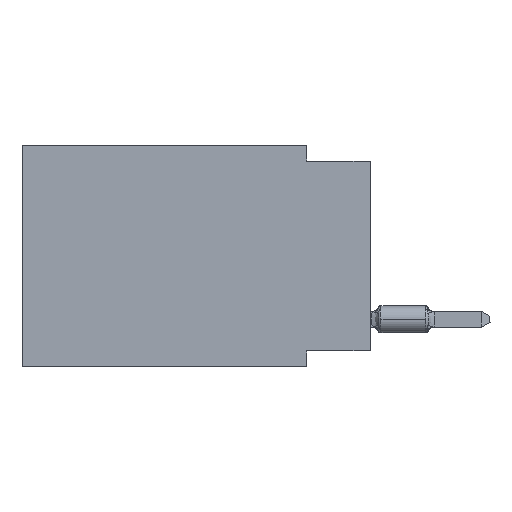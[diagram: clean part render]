
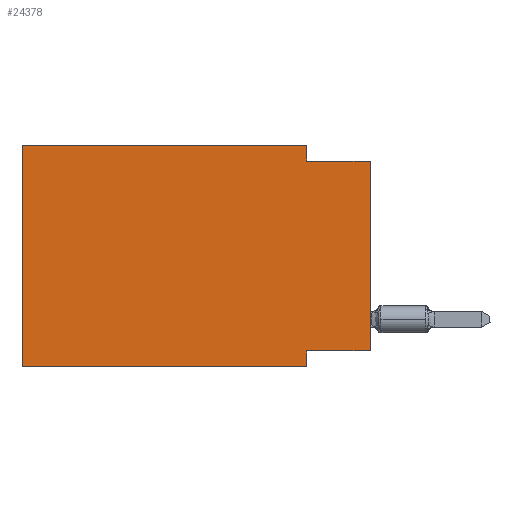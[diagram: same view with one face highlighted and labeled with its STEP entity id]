
A CAD part, left-side view. The second image highlights one B-rep face of the part: STEP entity #24378.
In plain terms, the highlighted planar face has unit normal (-1, 0, 0).
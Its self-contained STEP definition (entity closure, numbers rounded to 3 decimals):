
#668 = CARTESIAN_POINT ( 'NONE',  ( 0., 0., 0. ) ) ;
#763 = VECTOR ( 'NONE', #11287, 1000. ) ;
#2521 = CARTESIAN_POINT ( 'NONE',  ( 0., 2.54, -0.635 ) ) ;
#2656 = CARTESIAN_POINT ( 'NONE',  ( 0., 2.54, 0. ) ) ;
#3002 = DIRECTION ( 'NONE',  ( 0., 0., 1. ) ) ;
#3403 = DIRECTION ( 'NONE',  ( 0., -1., 0. ) ) ;
#3644 = EDGE_CURVE ( 'NONE', #13062, #7990, #9696, .T. ) ;
#3653 = LINE ( 'NONE', #25619, #9620 ) ;
#4362 = VERTEX_POINT ( 'NONE', #22403 ) ;
#4549 = DIRECTION ( 'NONE',  ( 0., 0., 1. ) ) ;
#5601 = LINE ( 'NONE', #14539, #17971 ) ;
#6176 = VERTEX_POINT ( 'NONE', #28338 ) ;
#6414 = DIRECTION ( 'NONE',  ( 0., -1., 0. ) ) ;
#6624 = LINE ( 'NONE', #9249, #17057 ) ;
#6654 = ORIENTED_EDGE ( 'NONE', *, *, #24984, .F. ) ;
#7820 = EDGE_CURVE ( 'NONE', #14424, #12782, #5601, .T. ) ;
#7990 = VERTEX_POINT ( 'NONE', #2521 ) ;
#9069 = CARTESIAN_POINT ( 'NONE',  ( 0., 13.97, 0. ) ) ;
#9249 = CARTESIAN_POINT ( 'NONE',  ( 0., 13.97, 0. ) ) ;
#9466 = LINE ( 'NONE', #668, #21795 ) ;
#9509 = ORIENTED_EDGE ( 'NONE', *, *, #7820, .F. ) ;
#9607 = EDGE_LOOP ( 'NONE', ( #22458, #11606, #20179, #6654, #10444, #12273, #9509, #18789 ) ) ;
#9620 = VECTOR ( 'NONE', #25482, 1000. ) ;
#9696 = LINE ( 'NONE', #2656, #17703 ) ;
#10444 = ORIENTED_EDGE ( 'NONE', *, *, #23944, .F. ) ;
#10953 = CARTESIAN_POINT ( 'NONE',  ( 0., 13.97, -8.89 ) ) ;
#11287 = DIRECTION ( 'NONE',  ( 0., 1., 0. ) ) ;
#11411 = DIRECTION ( 'NONE',  ( 1., 0., 0. ) ) ;
#11452 = DIRECTION ( 'NONE',  ( 0., 0., -1. ) ) ;
#11606 = ORIENTED_EDGE ( 'NONE', *, *, #23545, .F. ) ;
#12273 = ORIENTED_EDGE ( 'NONE', *, *, #27142, .T. ) ;
#12782 = VERTEX_POINT ( 'NONE', #22740 ) ;
#13062 = VERTEX_POINT ( 'NONE', #21847 ) ;
#13193 = CARTESIAN_POINT ( 'NONE',  ( 0., 0., -8.255 ) ) ;
#13339 = AXIS2_PLACEMENT_3D ( 'NONE', #9069, #11411, #20314 ) ;
#14209 = VERTEX_POINT ( 'NONE', #18851 ) ;
#14424 = VERTEX_POINT ( 'NONE', #16151 ) ;
#14539 = CARTESIAN_POINT ( 'NONE',  ( 0., 2.54, -8.89 ) ) ;
#14640 = VERTEX_POINT ( 'NONE', #24181 ) ;
#15621 = VECTOR ( 'NONE', #3403, 1000. ) ;
#16151 = CARTESIAN_POINT ( 'NONE',  ( 0., 2.54, -8.255 ) ) ;
#16248 = EDGE_CURVE ( 'NONE', #14209, #6176, #9466, .T. ) ;
#17057 = VECTOR ( 'NONE', #4549, 1000. ) ;
#17703 = VECTOR ( 'NONE', #11452, 1000. ) ;
#17771 = EDGE_CURVE ( 'NONE', #14209, #14424, #24301, .T. ) ;
#17971 = VECTOR ( 'NONE', #25512, 1000. ) ;
#18789 = ORIENTED_EDGE ( 'NONE', *, *, #17771, .F. ) ;
#18851 = CARTESIAN_POINT ( 'NONE',  ( 0., 0., -8.255 ) ) ;
#20171 = FACE_OUTER_BOUND ( 'NONE', #9607, .T. ) ;
#20179 = ORIENTED_EDGE ( 'NONE', *, *, #3644, .F. ) ;
#20314 = DIRECTION ( 'NONE',  ( 0., 0., -1. ) ) ;
#21795 = VECTOR ( 'NONE', #3002, 1000. ) ;
#21847 = CARTESIAN_POINT ( 'NONE',  ( 0., 2.54, 0. ) ) ;
#22403 = CARTESIAN_POINT ( 'NONE',  ( 0., 13.97, -8.89 ) ) ;
#22458 = ORIENTED_EDGE ( 'NONE', *, *, #16248, .T. ) ;
#22740 = CARTESIAN_POINT ( 'NONE',  ( 0., 2.54, -8.89 ) ) ;
#23545 = EDGE_CURVE ( 'NONE', #7990, #6176, #25211, .T. ) ;
#23944 = EDGE_CURVE ( 'NONE', #4362, #14640, #6624, .T. ) ;
#24181 = CARTESIAN_POINT ( 'NONE',  ( 0., 13.97, 0. ) ) ;
#24301 = LINE ( 'NONE', #13193, #763 ) ;
#24378 = ADVANCED_FACE ( 'NONE', ( #20171 ), #26897, .F. ) ;
#24984 = EDGE_CURVE ( 'NONE', #14640, #13062, #3653, .T. ) ;
#25211 = LINE ( 'NONE', #27686, #15621 ) ;
#25482 = DIRECTION ( 'NONE',  ( 0., -1., 0. ) ) ;
#25512 = DIRECTION ( 'NONE',  ( 0., 0., -1. ) ) ;
#25619 = CARTESIAN_POINT ( 'NONE',  ( 0., 13.97, 0. ) ) ;
#26447 = LINE ( 'NONE', #10953, #27068 ) ;
#26897 = PLANE ( 'NONE',  #13339 ) ;
#27068 = VECTOR ( 'NONE', #6414, 1000. ) ;
#27142 = EDGE_CURVE ( 'NONE', #4362, #12782, #26447, .T. ) ;
#27686 = CARTESIAN_POINT ( 'NONE',  ( 0., 0., -0.635 ) ) ;
#28338 = CARTESIAN_POINT ( 'NONE',  ( 0., 0., -0.635 ) ) ;
